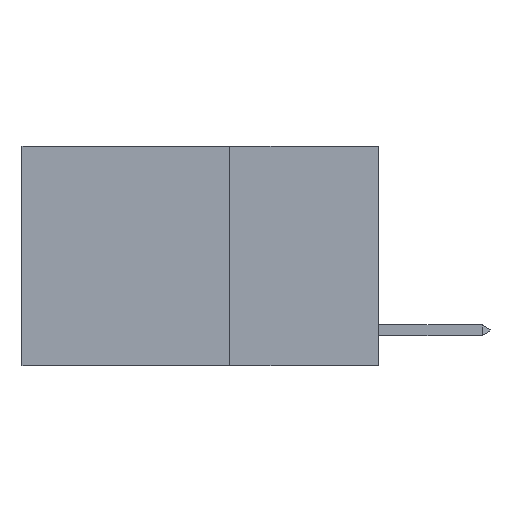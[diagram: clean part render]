
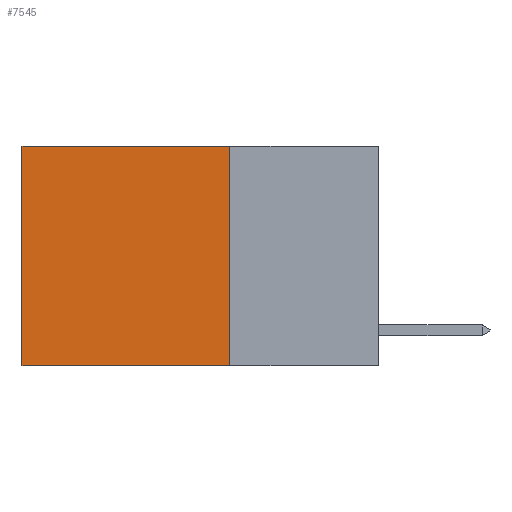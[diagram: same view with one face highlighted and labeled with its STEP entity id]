
A CAD part, left-side view. The second image highlights one B-rep face of the part: STEP entity #7545.
In plain terms, the highlighted planar face has unit normal (-1, 0, 0).
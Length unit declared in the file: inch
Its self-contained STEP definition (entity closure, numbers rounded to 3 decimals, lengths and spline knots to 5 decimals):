
#667 = CARTESIAN_POINT ( 'NONE',  ( 0.2625, 0.25, -0.37 ) ) ;
#1774 = LINE ( 'NONE', #11077, #2675 ) ;
#1916 = LINE ( 'NONE', #9608, #6041 ) ;
#2395 = EDGE_CURVE ( 'NONE', #9193, #10157, #6507, .T. ) ;
#2587 = PLANE ( 'NONE',  #12880 ) ;
#2675 = VECTOR ( 'NONE', #6991, 39.37008 ) ;
#2715 = CARTESIAN_POINT ( 'NONE',  ( 0.2625, 0.25, 0. ) ) ;
#2731 = VERTEX_POINT ( 'NONE', #667 ) ;
#3710 = VERTEX_POINT ( 'NONE', #11457 ) ;
#4080 = DIRECTION ( 'NONE',  ( 0., 0., -1. ) ) ;
#5553 = CARTESIAN_POINT ( 'NONE',  ( 0.2625, 0.25, -0.37 ) ) ;
#6041 = VECTOR ( 'NONE', #8228, 39.37008 ) ;
#6157 = FACE_OUTER_BOUND ( 'NONE', #16637, .T. ) ;
#6507 = LINE ( 'NONE', #2715, #13273 ) ;
#6991 = DIRECTION ( 'NONE',  ( 0., 0., -1. ) ) ;
#7545 = ADVANCED_FACE ( 'NONE', ( #6157 ), #2587, .F. ) ;
#8166 = ORIENTED_EDGE ( 'NONE', *, *, #16751, .F. ) ;
#8228 = DIRECTION ( 'NONE',  ( 0., 0., -1. ) ) ;
#8275 = EDGE_CURVE ( 'NONE', #10157, #3710, #1774, .T. ) ;
#8350 = VECTOR ( 'NONE', #9650, 39.37008 ) ;
#9193 = VERTEX_POINT ( 'NONE', #13007 ) ;
#9547 = ORIENTED_EDGE ( 'NONE', *, *, #16047, .F. ) ;
#9608 = CARTESIAN_POINT ( 'NONE',  ( 0.2625, 0.25, 0. ) ) ;
#9650 = DIRECTION ( 'NONE',  ( 0., 1., 0. ) ) ;
#10157 = VERTEX_POINT ( 'NONE', #12538 ) ;
#10826 = ORIENTED_EDGE ( 'NONE', *, *, #2395, .T. ) ;
#10853 = CARTESIAN_POINT ( 'NONE',  ( 0.2625, 0.25, 0. ) ) ;
#11077 = CARTESIAN_POINT ( 'NONE',  ( 0.2625, 0.6, 0. ) ) ;
#11457 = CARTESIAN_POINT ( 'NONE',  ( 0.2625, 0.6, -0.37 ) ) ;
#11963 = LINE ( 'NONE', #5553, #8350 ) ;
#12048 = ORIENTED_EDGE ( 'NONE', *, *, #8275, .T. ) ;
#12226 = DIRECTION ( 'NONE',  ( 1., 0., 0. ) ) ;
#12286 = DIRECTION ( 'NONE',  ( 0., 1., 0. ) ) ;
#12538 = CARTESIAN_POINT ( 'NONE',  ( 0.2625, 0.6, 0. ) ) ;
#12880 = AXIS2_PLACEMENT_3D ( 'NONE', #10853, #12226, #4080 ) ;
#13007 = CARTESIAN_POINT ( 'NONE',  ( 0.2625, 0.25, 0. ) ) ;
#13273 = VECTOR ( 'NONE', #12286, 39.37008 ) ;
#16047 = EDGE_CURVE ( 'NONE', #9193, #2731, #1916, .T. ) ;
#16637 = EDGE_LOOP ( 'NONE', ( #12048, #8166, #9547, #10826 ) ) ;
#16751 = EDGE_CURVE ( 'NONE', #2731, #3710, #11963, .T. ) ;
